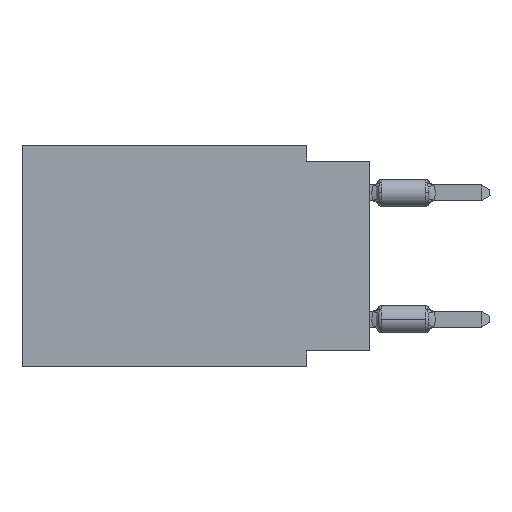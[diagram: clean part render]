
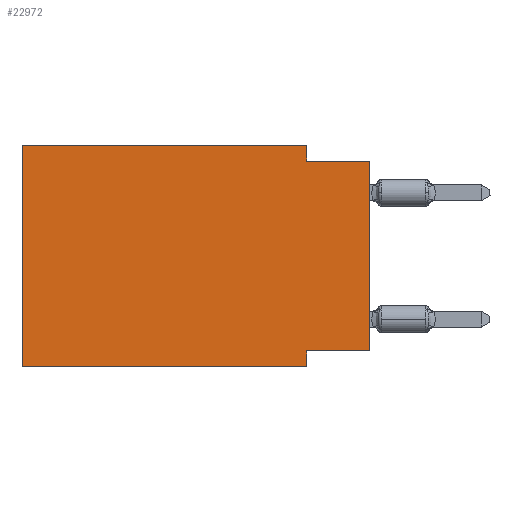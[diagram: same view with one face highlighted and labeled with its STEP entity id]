
A CAD part, left-side view. The second image highlights one B-rep face of the part: STEP entity #22972.
In plain terms, the highlighted planar face has unit normal (-1, 0, 0).
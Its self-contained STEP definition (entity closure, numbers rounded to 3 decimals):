
#54 = DIRECTION ( 'NONE',  ( 0., -1., 0. ) ) ;
#1015 = VERTEX_POINT ( 'NONE', #21300 ) ;
#1413 = ORIENTED_EDGE ( 'NONE', *, *, #26991, .T. ) ;
#1800 = LINE ( 'NONE', #18658, #24507 ) ;
#1993 = ORIENTED_EDGE ( 'NONE', *, *, #29611, .F. ) ;
#2491 = VECTOR ( 'NONE', #32717, 1000. ) ;
#2623 = LINE ( 'NONE', #24140, #2491 ) ;
#3454 = LINE ( 'NONE', #24636, #15316 ) ;
#3833 = EDGE_CURVE ( 'NONE', #14285, #24879, #15067, .T. ) ;
#3836 = VERTEX_POINT ( 'NONE', #4301 ) ;
#4065 = DIRECTION ( 'NONE',  ( 0., 0., 1. ) ) ;
#4301 = CARTESIAN_POINT ( 'NONE',  ( 0., 0., -0.635 ) ) ;
#4630 = ORIENTED_EDGE ( 'NONE', *, *, #26367, .T. ) ;
#5860 = CARTESIAN_POINT ( 'NONE',  ( 0., 13.97, 0. ) ) ;
#6300 = LINE ( 'NONE', #17249, #19730 ) ;
#6417 = VERTEX_POINT ( 'NONE', #33258 ) ;
#6678 = DIRECTION ( 'NONE',  ( 1., 0., 0. ) ) ;
#6925 = LINE ( 'NONE', #12130, #13639 ) ;
#8136 = CARTESIAN_POINT ( 'NONE',  ( 0., 2.54, -8.89 ) ) ;
#8315 = LINE ( 'NONE', #8136, #9921 ) ;
#9160 = VERTEX_POINT ( 'NONE', #27666 ) ;
#9463 = VECTOR ( 'NONE', #11251, 1000. ) ;
#9921 = VECTOR ( 'NONE', #13536, 1000. ) ;
#10653 = EDGE_LOOP ( 'NONE', ( #1413, #1993, #19729, #25700, #21892, #4630, #33660, #17625 ) ) ;
#10910 = LINE ( 'NONE', #18821, #9463 ) ;
#11141 = EDGE_CURVE ( 'NONE', #6417, #9160, #8315, .T. ) ;
#11251 = DIRECTION ( 'NONE',  ( 0., -1., 0. ) ) ;
#11709 = EDGE_CURVE ( 'NONE', #24879, #1015, #6300, .T. ) ;
#12130 = CARTESIAN_POINT ( 'NONE',  ( 0., 13.97, 0. ) ) ;
#12373 = DIRECTION ( 'NONE',  ( 0., -1., 0. ) ) ;
#12729 = DIRECTION ( 'NONE',  ( 0., 1., 0. ) ) ;
#13536 = DIRECTION ( 'NONE',  ( 0., 0., -1. ) ) ;
#13639 = VECTOR ( 'NONE', #4065, 1000. ) ;
#13880 = AXIS2_PLACEMENT_3D ( 'NONE', #28544, #6678, #17626 ) ;
#14285 = VERTEX_POINT ( 'NONE', #5860 ) ;
#15067 = LINE ( 'NONE', #26014, #22531 ) ;
#15316 = VECTOR ( 'NONE', #54, 1000. ) ;
#17212 = EDGE_CURVE ( 'NONE', #22610, #6417, #1800, .T. ) ;
#17249 = CARTESIAN_POINT ( 'NONE',  ( 0., 2.54, 0. ) ) ;
#17625 = ORIENTED_EDGE ( 'NONE', *, *, #17212, .F. ) ;
#17626 = DIRECTION ( 'NONE',  ( 0., 0., -1. ) ) ;
#17919 = EDGE_CURVE ( 'NONE', #27475, #14285, #6925, .T. ) ;
#18658 = CARTESIAN_POINT ( 'NONE',  ( 0., 0., -8.255 ) ) ;
#18821 = CARTESIAN_POINT ( 'NONE',  ( 0., 0., -0.635 ) ) ;
#19729 = ORIENTED_EDGE ( 'NONE', *, *, #11709, .F. ) ;
#19730 = VECTOR ( 'NONE', #28162, 1000. ) ;
#20321 = FACE_OUTER_BOUND ( 'NONE', #10653, .T. ) ;
#21300 = CARTESIAN_POINT ( 'NONE',  ( 0., 2.54, -0.635 ) ) ;
#21892 = ORIENTED_EDGE ( 'NONE', *, *, #17919, .F. ) ;
#22531 = VECTOR ( 'NONE', #12373, 1000. ) ;
#22610 = VERTEX_POINT ( 'NONE', #24467 ) ;
#22972 = ADVANCED_FACE ( 'NONE', ( #20321 ), #31224, .F. ) ;
#24140 = CARTESIAN_POINT ( 'NONE',  ( 0., 0., 0. ) ) ;
#24467 = CARTESIAN_POINT ( 'NONE',  ( 0., 0., -8.255 ) ) ;
#24507 = VECTOR ( 'NONE', #12729, 1000. ) ;
#24636 = CARTESIAN_POINT ( 'NONE',  ( 0., 13.97, -8.89 ) ) ;
#24879 = VERTEX_POINT ( 'NONE', #35412 ) ;
#25700 = ORIENTED_EDGE ( 'NONE', *, *, #3833, .F. ) ;
#26014 = CARTESIAN_POINT ( 'NONE',  ( 0., 13.97, 0. ) ) ;
#26367 = EDGE_CURVE ( 'NONE', #27475, #9160, #3454, .T. ) ;
#26991 = EDGE_CURVE ( 'NONE', #22610, #3836, #2623, .T. ) ;
#27475 = VERTEX_POINT ( 'NONE', #33563 ) ;
#27666 = CARTESIAN_POINT ( 'NONE',  ( 0., 2.54, -8.89 ) ) ;
#28162 = DIRECTION ( 'NONE',  ( 0., 0., -1. ) ) ;
#28544 = CARTESIAN_POINT ( 'NONE',  ( 0., 13.97, 0. ) ) ;
#29611 = EDGE_CURVE ( 'NONE', #1015, #3836, #10910, .T. ) ;
#31224 = PLANE ( 'NONE',  #13880 ) ;
#32717 = DIRECTION ( 'NONE',  ( 0., 0., 1. ) ) ;
#33258 = CARTESIAN_POINT ( 'NONE',  ( 0., 2.54, -8.255 ) ) ;
#33563 = CARTESIAN_POINT ( 'NONE',  ( 0., 13.97, -8.89 ) ) ;
#33660 = ORIENTED_EDGE ( 'NONE', *, *, #11141, .F. ) ;
#35412 = CARTESIAN_POINT ( 'NONE',  ( 0., 2.54, 0. ) ) ;
